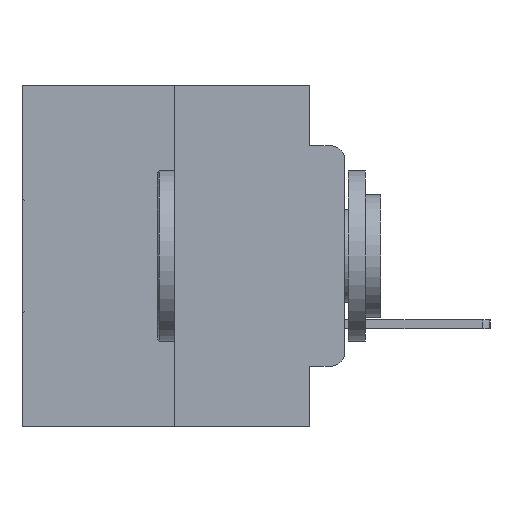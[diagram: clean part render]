
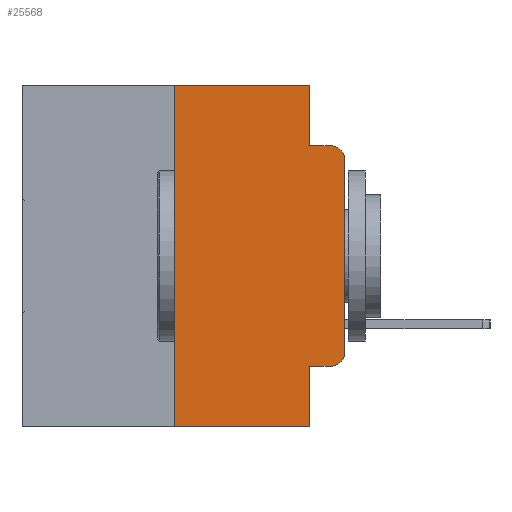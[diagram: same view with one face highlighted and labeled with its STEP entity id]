
A CAD part, left-side view. The second image highlights one B-rep face of the part: STEP entity #25568.
In plain terms, the highlighted planar face has unit normal (-1, 0, 0).
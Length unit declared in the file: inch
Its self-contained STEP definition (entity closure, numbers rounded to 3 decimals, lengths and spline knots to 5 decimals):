
#222 = DIRECTION ( 'NONE',  ( 0., 0., -1. ) ) ;
#804 = VECTOR ( 'NONE', #17889, 39.37008 ) ;
#806 = DIRECTION ( 'NONE',  ( 0., 0., -1. ) ) ;
#2413 = ORIENTED_EDGE ( 'NONE', *, *, #2899, .T. ) ;
#2671 = CARTESIAN_POINT ( 'NONE',  ( 0., 0.473, -0.5 ) ) ;
#2867 = CARTESIAN_POINT ( 'NONE',  ( 0., 0., -0.1085 ) ) ;
#2899 = EDGE_CURVE ( 'NONE', #14939, #16417, #10374, .T. ) ;
#2985 = LINE ( 'NONE', #27770, #25782 ) ;
#3458 = VECTOR ( 'NONE', #6015, 39.37008 ) ;
#5110 = VECTOR ( 'NONE', #5197, 39.37008 ) ;
#5197 = DIRECTION ( 'NONE',  ( 0., -1., 0. ) ) ;
#5371 = VECTOR ( 'NONE', #13119, 39.37008 ) ;
#5613 = EDGE_CURVE ( 'NONE', #12310, #13986, #18830, .T. ) ;
#6015 = DIRECTION ( 'NONE',  ( 0., -1., 0. ) ) ;
#6398 = ORIENTED_EDGE ( 'NONE', *, *, #17470, .T. ) ;
#6845 = CARTESIAN_POINT ( 'NONE',  ( 0., 0.051, 0. ) ) ;
#6941 = VERTEX_POINT ( 'NONE', #7561 ) ;
#7048 = LINE ( 'NONE', #6845, #804 ) ;
#7120 = ORIENTED_EDGE ( 'NONE', *, *, #14514, .F. ) ;
#7561 = CARTESIAN_POINT ( 'NONE',  ( 0., 0.051, 0. ) ) ;
#7789 = ORIENTED_EDGE ( 'NONE', *, *, #11596, .F. ) ;
#7855 = CARTESIAN_POINT ( 'NONE',  ( 0., 0.473, 0. ) ) ;
#8219 = DIRECTION ( 'NONE',  ( 0., -1., 0. ) ) ;
#8644 = EDGE_CURVE ( 'NONE', #24032, #12310, #2985, .T. ) ;
#10093 = DIRECTION ( 'NONE',  ( 0., 0., -1. ) ) ;
#10122 = EDGE_CURVE ( 'NONE', #24032, #16417, #26724, .T. ) ;
#10193 = LINE ( 'NONE', #17000, #3458 ) ;
#10223 = EDGE_LOOP ( 'NONE', ( #28261, #6398, #18111, #7120, #18762, #7789, #2413, #25915, #15715, #16384 ) ) ;
#10374 = LINE ( 'NONE', #2671, #5110 ) ;
#11210 = CIRCLE ( 'NONE', #25267, 0.02 ) ;
#11596 = EDGE_CURVE ( 'NONE', #14939, #22958, #12712, .T. ) ;
#12042 = DIRECTION ( 'NONE',  ( 0., -1., 0. ) ) ;
#12310 = VERTEX_POINT ( 'NONE', #18243 ) ;
#12712 = LINE ( 'NONE', #26243, #5371 ) ;
#12794 = VECTOR ( 'NONE', #24974, 39.37008 ) ;
#13119 = DIRECTION ( 'NONE',  ( 0., 0., 1. ) ) ;
#13813 = EDGE_CURVE ( 'NONE', #22958, #6941, #10193, .T. ) ;
#13816 = DIRECTION ( 'NONE',  ( -1., 0., 0. ) ) ;
#13826 = VECTOR ( 'NONE', #12042, 39.37008 ) ;
#13986 = VERTEX_POINT ( 'NONE', #21943 ) ;
#14344 = DIRECTION ( 'NONE',  ( -1., 0., 0. ) ) ;
#14514 = EDGE_CURVE ( 'NONE', #6941, #15708, #7048, .T. ) ;
#14939 = VERTEX_POINT ( 'NONE', #23652 ) ;
#15134 = VECTOR ( 'NONE', #17661, 39.37008 ) ;
#15708 = VERTEX_POINT ( 'NONE', #21898 ) ;
#15715 = ORIENTED_EDGE ( 'NONE', *, *, #8644, .T. ) ;
#16004 = EDGE_CURVE ( 'NONE', #15708, #25287, #25398, .T. ) ;
#16384 = ORIENTED_EDGE ( 'NONE', *, *, #5613, .T. ) ;
#16417 = VERTEX_POINT ( 'NONE', #28654 ) ;
#16916 = CARTESIAN_POINT ( 'NONE',  ( 0., 0.051, -0.4115 ) ) ;
#17000 = CARTESIAN_POINT ( 'NONE',  ( 0., 0.473, 0. ) ) ;
#17470 = EDGE_CURVE ( 'NONE', #18694, #25287, #11210, .T. ) ;
#17661 = DIRECTION ( 'NONE',  ( 0., 0., -1. ) ) ;
#17889 = DIRECTION ( 'NONE',  ( 0., 0., -1. ) ) ;
#18111 = ORIENTED_EDGE ( 'NONE', *, *, #16004, .F. ) ;
#18243 = CARTESIAN_POINT ( 'NONE',  ( 0., 0.02, -0.4115 ) ) ;
#18694 = VERTEX_POINT ( 'NONE', #2867 ) ;
#18762 = ORIENTED_EDGE ( 'NONE', *, *, #13813, .F. ) ;
#18830 = CIRCLE ( 'NONE', #20655, 0.02 ) ;
#20163 = AXIS2_PLACEMENT_3D ( 'NONE', #7855, #23162, #10093 ) ;
#20372 = EDGE_CURVE ( 'NONE', #13986, #18694, #24401, .T. ) ;
#20655 = AXIS2_PLACEMENT_3D ( 'NONE', #27365, #14344, #806 ) ;
#20970 = PLANE ( 'NONE',  #20163 ) ;
#21898 = CARTESIAN_POINT ( 'NONE',  ( 0., 0.051, -0.0885 ) ) ;
#21943 = CARTESIAN_POINT ( 'NONE',  ( 0., 0., -0.3915 ) ) ;
#22958 = VERTEX_POINT ( 'NONE', #23942 ) ;
#23162 = DIRECTION ( 'NONE',  ( 1., 0., 0. ) ) ;
#23652 = CARTESIAN_POINT ( 'NONE',  ( 0., 0.25, -0.5 ) ) ;
#23942 = CARTESIAN_POINT ( 'NONE',  ( 0., 0.25, 0. ) ) ;
#24001 = CARTESIAN_POINT ( 'NONE',  ( 0., 0.02, -0.0885 ) ) ;
#24032 = VERTEX_POINT ( 'NONE', #16916 ) ;
#24122 = CARTESIAN_POINT ( 'NONE',  ( 0., 0.051, 0. ) ) ;
#24401 = LINE ( 'NONE', #27136, #12794 ) ;
#24974 = DIRECTION ( 'NONE',  ( 0., 0., 1. ) ) ;
#25096 = CARTESIAN_POINT ( 'NONE',  ( 0., 0.051, -0.0885 ) ) ;
#25267 = AXIS2_PLACEMENT_3D ( 'NONE', #26856, #13816, #222 ) ;
#25287 = VERTEX_POINT ( 'NONE', #24001 ) ;
#25398 = LINE ( 'NONE', #25096, #13826 ) ;
#25568 = ADVANCED_FACE ( 'NONE', ( #27499 ), #20970, .F. ) ;
#25782 = VECTOR ( 'NONE', #8219, 39.37008 ) ;
#25915 = ORIENTED_EDGE ( 'NONE', *, *, #10122, .F. ) ;
#26243 = CARTESIAN_POINT ( 'NONE',  ( 0., 0.25, 0. ) ) ;
#26724 = LINE ( 'NONE', #24122, #15134 ) ;
#26856 = CARTESIAN_POINT ( 'NONE',  ( 0., 0.02, -0.1085 ) ) ;
#27136 = CARTESIAN_POINT ( 'NONE',  ( 0., 0., 0. ) ) ;
#27365 = CARTESIAN_POINT ( 'NONE',  ( 0., 0.02, -0.3915 ) ) ;
#27499 = FACE_OUTER_BOUND ( 'NONE', #10223, .T. ) ;
#27770 = CARTESIAN_POINT ( 'NONE',  ( 0., 0.051, -0.4115 ) ) ;
#28261 = ORIENTED_EDGE ( 'NONE', *, *, #20372, .T. ) ;
#28654 = CARTESIAN_POINT ( 'NONE',  ( 0., 0.051, -0.5 ) ) ;
